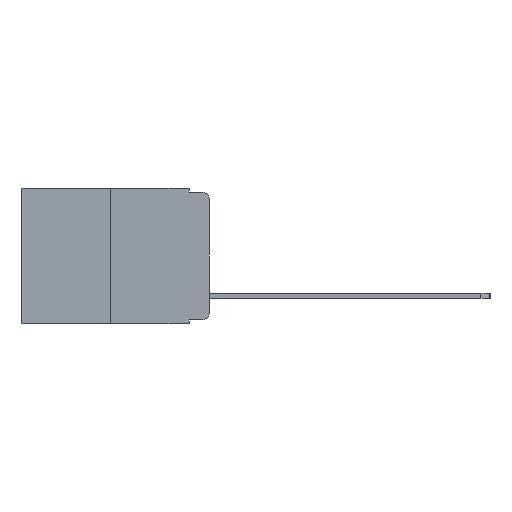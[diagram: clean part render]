
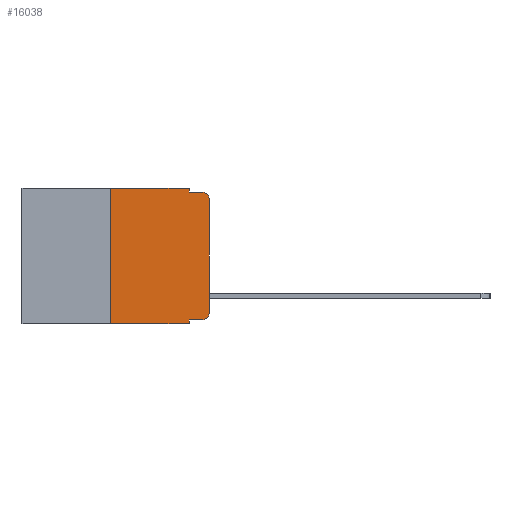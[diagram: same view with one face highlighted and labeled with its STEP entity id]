
A CAD part, left-side view. The second image highlights one B-rep face of the part: STEP entity #16038.
In plain terms, the highlighted planar face has unit normal (-1, 0, 0).
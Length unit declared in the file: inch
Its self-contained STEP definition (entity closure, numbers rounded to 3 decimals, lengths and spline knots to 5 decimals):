
#204 = VERTEX_POINT ( 'NONE', #11136 ) ;
#252 = ORIENTED_EDGE ( 'NONE', *, *, #4160, .F. ) ;
#344 = VECTOR ( 'NONE', #5421, 39.37008 ) ;
#609 = CARTESIAN_POINT ( 'NONE',  ( 0., 0.051, -0.333 ) ) ;
#896 = EDGE_CURVE ( 'NONE', #15945, #4992, #16090, .T. ) ;
#1213 = CARTESIAN_POINT ( 'NONE',  ( 0., 0.473, 0. ) ) ;
#1419 = DIRECTION ( 'NONE',  ( 0., 0., 1. ) ) ;
#1422 = CARTESIAN_POINT ( 'NONE',  ( 0., 0., -0.03 ) ) ;
#2114 = DIRECTION ( 'NONE',  ( 0., -1., 0. ) ) ;
#2211 = LINE ( 'NONE', #2887, #6428 ) ;
#2362 = VERTEX_POINT ( 'NONE', #10366 ) ;
#2887 = CARTESIAN_POINT ( 'NONE',  ( 0., 0.051, 0. ) ) ;
#3495 = DIRECTION ( 'NONE',  ( 0., -1., 0. ) ) ;
#3664 = LINE ( 'NONE', #15594, #11275 ) ;
#4090 = ORIENTED_EDGE ( 'NONE', *, *, #14094, .T. ) ;
#4095 = CARTESIAN_POINT ( 'NONE',  ( 0., 0., 0. ) ) ;
#4160 = EDGE_CURVE ( 'NONE', #14934, #18046, #5347, .T. ) ;
#4169 = VERTEX_POINT ( 'NONE', #14531 ) ;
#4290 = EDGE_LOOP ( 'NONE', ( #19452, #4090, #252, #4598, #5111, #13038, #16920, #13956, #14404, #18341 ) ) ;
#4598 = ORIENTED_EDGE ( 'NONE', *, *, #9308, .F. ) ;
#4846 = EDGE_CURVE ( 'NONE', #17611, #4169, #6300, .T. ) ;
#4992 = VERTEX_POINT ( 'NONE', #1422 ) ;
#5000 = LINE ( 'NONE', #19442, #12937 ) ;
#5111 = ORIENTED_EDGE ( 'NONE', *, *, #8973, .F. ) ;
#5347 = LINE ( 'NONE', #14567, #8902 ) ;
#5421 = DIRECTION ( 'NONE',  ( 0., 0., 1. ) ) ;
#5736 = VERTEX_POINT ( 'NONE', #18850 ) ;
#5983 = CARTESIAN_POINT ( 'NONE',  ( 0., 0.02, -0.313 ) ) ;
#5988 = PLANE ( 'NONE',  #18268 ) ;
#6056 = DIRECTION ( 'NONE',  ( 0., 0., -1. ) ) ;
#6300 = LINE ( 'NONE', #17467, #14140 ) ;
#6428 = VECTOR ( 'NONE', #14895, 39.37008 ) ;
#6815 = CARTESIAN_POINT ( 'NONE',  ( 0., 0.473, 0. ) ) ;
#6957 = CARTESIAN_POINT ( 'NONE',  ( 0., 0., -0.313 ) ) ;
#7495 = DIRECTION ( 'NONE',  ( -1., 0., 0. ) ) ;
#7534 = DIRECTION ( 'NONE',  ( 0., 0., -1. ) ) ;
#7853 = EDGE_CURVE ( 'NONE', #11498, #15945, #18231, .T. ) ;
#7967 = EDGE_CURVE ( 'NONE', #5736, #2362, #5000, .T. ) ;
#8902 = VECTOR ( 'NONE', #10605, 39.37008 ) ;
#8973 = EDGE_CURVE ( 'NONE', #2362, #204, #19317, .T. ) ;
#9281 = AXIS2_PLACEMENT_3D ( 'NONE', #16260, #7495, #17740 ) ;
#9308 = EDGE_CURVE ( 'NONE', #204, #14934, #2211, .T. ) ;
#9331 = VECTOR ( 'NONE', #3495, 39.37008 ) ;
#10190 = DIRECTION ( 'NONE',  ( 0., 0., -1. ) ) ;
#10199 = EDGE_CURVE ( 'NONE', #17611, #11498, #3664, .T. ) ;
#10366 = CARTESIAN_POINT ( 'NONE',  ( 0., 0.25, 0. ) ) ;
#10605 = DIRECTION ( 'NONE',  ( 0., -1., 0. ) ) ;
#11136 = CARTESIAN_POINT ( 'NONE',  ( 0., 0.051, 0. ) ) ;
#11275 = VECTOR ( 'NONE', #17089, 39.37008 ) ;
#11498 = VERTEX_POINT ( 'NONE', #15551 ) ;
#11719 = CIRCLE ( 'NONE', #9281, 0.02 ) ;
#12160 = AXIS2_PLACEMENT_3D ( 'NONE', #5983, #16297, #7534 ) ;
#12536 = CARTESIAN_POINT ( 'NONE',  ( 0., 0.473, -0.343 ) ) ;
#12642 = EDGE_CURVE ( 'NONE', #5736, #4169, #13679, .T. ) ;
#12937 = VECTOR ( 'NONE', #1419, 39.37008 ) ;
#13030 = FACE_OUTER_BOUND ( 'NONE', #4290, .T. ) ;
#13038 = ORIENTED_EDGE ( 'NONE', *, *, #7967, .F. ) ;
#13679 = LINE ( 'NONE', #12536, #9331 ) ;
#13956 = ORIENTED_EDGE ( 'NONE', *, *, #4846, .F. ) ;
#14094 = EDGE_CURVE ( 'NONE', #4992, #18046, #11719, .T. ) ;
#14140 = VECTOR ( 'NONE', #10190, 39.37008 ) ;
#14404 = ORIENTED_EDGE ( 'NONE', *, *, #10199, .T. ) ;
#14531 = CARTESIAN_POINT ( 'NONE',  ( 0., 0.051, -0.343 ) ) ;
#14567 = CARTESIAN_POINT ( 'NONE',  ( 0., 0.051, -0.01 ) ) ;
#14888 = DIRECTION ( 'NONE',  ( 1., 0., 0. ) ) ;
#14895 = DIRECTION ( 'NONE',  ( 0., 0., -1. ) ) ;
#14934 = VERTEX_POINT ( 'NONE', #19498 ) ;
#15318 = CARTESIAN_POINT ( 'NONE',  ( 0., 0.02, -0.01 ) ) ;
#15399 = VECTOR ( 'NONE', #2114, 39.37008 ) ;
#15551 = CARTESIAN_POINT ( 'NONE',  ( 0., 0.02, -0.333 ) ) ;
#15594 = CARTESIAN_POINT ( 'NONE',  ( 0., 0.051, -0.333 ) ) ;
#15945 = VERTEX_POINT ( 'NONE', #6957 ) ;
#16038 = ADVANCED_FACE ( 'NONE', ( #13030 ), #5988, .F. ) ;
#16090 = LINE ( 'NONE', #4095, #344 ) ;
#16260 = CARTESIAN_POINT ( 'NONE',  ( 0., 0.02, -0.03 ) ) ;
#16297 = DIRECTION ( 'NONE',  ( -1., 0., 0. ) ) ;
#16920 = ORIENTED_EDGE ( 'NONE', *, *, #12642, .T. ) ;
#17089 = DIRECTION ( 'NONE',  ( 0., -1., 0. ) ) ;
#17467 = CARTESIAN_POINT ( 'NONE',  ( 0., 0.051, 0. ) ) ;
#17611 = VERTEX_POINT ( 'NONE', #609 ) ;
#17740 = DIRECTION ( 'NONE',  ( 0., 0., -1. ) ) ;
#18046 = VERTEX_POINT ( 'NONE', #15318 ) ;
#18231 = CIRCLE ( 'NONE', #12160, 0.02 ) ;
#18268 = AXIS2_PLACEMENT_3D ( 'NONE', #1213, #14888, #6056 ) ;
#18341 = ORIENTED_EDGE ( 'NONE', *, *, #7853, .T. ) ;
#18850 = CARTESIAN_POINT ( 'NONE',  ( 0., 0.25, -0.343 ) ) ;
#19317 = LINE ( 'NONE', #6815, #15399 ) ;
#19442 = CARTESIAN_POINT ( 'NONE',  ( 0., 0.25, 0. ) ) ;
#19452 = ORIENTED_EDGE ( 'NONE', *, *, #896, .T. ) ;
#19498 = CARTESIAN_POINT ( 'NONE',  ( 0., 0.051, -0.01 ) ) ;
